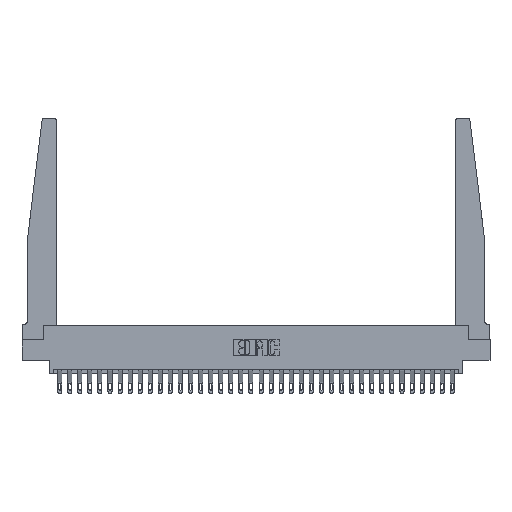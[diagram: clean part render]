
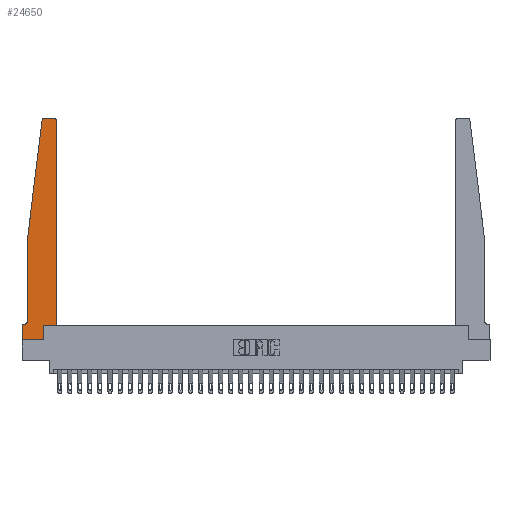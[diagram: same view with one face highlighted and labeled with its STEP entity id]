
A CAD part, top view. The second image highlights one B-rep face of the part: STEP entity #24650.
In plain terms, the highlighted planar face has unit normal (0, 0, 1).
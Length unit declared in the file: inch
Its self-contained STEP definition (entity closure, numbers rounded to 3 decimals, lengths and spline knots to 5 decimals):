
#152 = DIRECTION ( 'NONE',  ( 1., 0., 0. ) ) ;
#312 = PLANE ( 'NONE',  #7482 ) ;
#582 = CARTESIAN_POINT ( 'NONE',  ( 0.065, 1.25, 0.37 ) ) ;
#1792 = ORIENTED_EDGE ( 'NONE', *, *, #31335, .T. ) ;
#2020 = ORIENTED_EDGE ( 'NONE', *, *, #15700, .T. ) ;
#2259 = VECTOR ( 'NONE', #19090, 39.37008 ) ;
#2530 = DIRECTION ( 'NONE',  ( -1., 0., 0. ) ) ;
#2565 = VERTEX_POINT ( 'NONE', #5138 ) ;
#3708 = DIRECTION ( 'NONE',  ( 0., 0., 1. ) ) ;
#4409 = ORIENTED_EDGE ( 'NONE', *, *, #10294, .T. ) ;
#4906 = CIRCLE ( 'NONE', #15784, 0.03 ) ;
#4925 = EDGE_LOOP ( 'NONE', ( #30209, #31184, #9710, #9682, #20174, #4409, #19784, #1792, #2020, #24853, #12709, #20720 ) ) ;
#5138 = CARTESIAN_POINT ( 'NONE',  ( 0.2605, 0.18, 0.37 ) ) ;
#5586 = CARTESIAN_POINT ( 'NONE',  ( 0.425, 0.18, 0.37 ) ) ;
#5610 = CARTESIAN_POINT ( 'NONE',  ( 0.015, 0.2375, 0.37 ) ) ;
#5785 = DIRECTION ( 'NONE',  ( 0., -1., 0. ) ) ;
#7321 = CARTESIAN_POINT ( 'NONE',  ( 0., 0., 0.37 ) ) ;
#7384 = DIRECTION ( 'NONE',  ( 0., 1., 0. ) ) ;
#7482 = AXIS2_PLACEMENT_3D ( 'NONE', #13134, #24829, #152 ) ;
#7746 = VECTOR ( 'NONE', #2530, 39.37008 ) ;
#8170 = EDGE_CURVE ( 'NONE', #2565, #14448, #26695, .T. ) ;
#9081 = VERTEX_POINT ( 'NONE', #29151 ) ;
#9682 = ORIENTED_EDGE ( 'NONE', *, *, #30110, .T. ) ;
#9704 = EDGE_CURVE ( 'NONE', #14448, #24327, #17761, .T. ) ;
#9710 = ORIENTED_EDGE ( 'NONE', *, *, #24084, .T. ) ;
#9741 = EDGE_CURVE ( 'NONE', #17023, #22354, #15329, .T. ) ;
#9777 = VECTOR ( 'NONE', #9955, 39.37008 ) ;
#9955 = DIRECTION ( 'NONE',  ( 0., -1., 0. ) ) ;
#10294 = EDGE_CURVE ( 'NONE', #11463, #24770, #20957, .T. ) ;
#10529 = CARTESIAN_POINT ( 'NONE',  ( 0.24675, 2.72367, 0.37 ) ) ;
#10825 = CARTESIAN_POINT ( 'NONE',  ( 0.065, 1.25, 0.37 ) ) ;
#10858 = CARTESIAN_POINT ( 'NONE',  ( 0., 0.1875, 0.37 ) ) ;
#11349 = VECTOR ( 'NONE', #27652, 39.37008 ) ;
#11463 = VERTEX_POINT ( 'NONE', #30847 ) ;
#11515 = VECTOR ( 'NONE', #7384, 39.37008 ) ;
#11937 = DIRECTION ( 'NONE',  ( 0., 0., 1. ) ) ;
#11976 = CARTESIAN_POINT ( 'NONE',  ( 0., 0., 0.37 ) ) ;
#12094 = CARTESIAN_POINT ( 'NONE',  ( 0.395, 2.72, 0.37 ) ) ;
#12186 = DIRECTION ( 'NONE',  ( 1., 0., 0. ) ) ;
#12709 = ORIENTED_EDGE ( 'NONE', *, *, #9704, .T. ) ;
#13134 = CARTESIAN_POINT ( 'NONE',  ( 0., 0.1875, 0.37 ) ) ;
#13594 = AXIS2_PLACEMENT_3D ( 'NONE', #5610, #17783, #27669 ) ;
#13626 = DIRECTION ( 'NONE',  ( 1., 0., 0. ) ) ;
#14052 = DIRECTION ( 'NONE',  ( 1., 0., 0. ) ) ;
#14448 = VERTEX_POINT ( 'NONE', #26674 ) ;
#14480 = VECTOR ( 'NONE', #28961, 39.37008 ) ;
#14578 = EDGE_CURVE ( 'NONE', #24770, #17082, #29259, .T. ) ;
#15088 = FACE_OUTER_BOUND ( 'NONE', #4925, .T. ) ;
#15329 = LINE ( 'NONE', #24750, #7746 ) ;
#15700 = EDGE_CURVE ( 'NONE', #9081, #2565, #24905, .T. ) ;
#15784 = AXIS2_PLACEMENT_3D ( 'NONE', #12094, #11937, #14052 ) ;
#16792 = CARTESIAN_POINT ( 'NONE',  ( 0.425, 0.18, 0.37 ) ) ;
#16940 = CARTESIAN_POINT ( 'NONE',  ( 0., 0., 0.37 ) ) ;
#17023 = VERTEX_POINT ( 'NONE', #29014 ) ;
#17082 = VERTEX_POINT ( 'NONE', #11976 ) ;
#17761 = LINE ( 'NONE', #5586, #11349 ) ;
#17783 = DIRECTION ( 'NONE',  ( 0., 0., -1. ) ) ;
#17873 = EDGE_CURVE ( 'NONE', #26345, #11463, #24472, .T. ) ;
#18444 = CARTESIAN_POINT ( 'NONE',  ( 0.065, 0.2375, 0.37 ) ) ;
#18525 = CARTESIAN_POINT ( 'NONE',  ( 0.065, 0.1875, 0.37 ) ) ;
#18791 = CARTESIAN_POINT ( 'NONE',  ( 0.27653, 2.75, 0.37 ) ) ;
#18938 = EDGE_CURVE ( 'NONE', #22354, #28500, #23054, .T. ) ;
#19090 = DIRECTION ( 'NONE',  ( -0.122, -0.992, 0. ) ) ;
#19181 = LINE ( 'NONE', #7321, #20954 ) ;
#19784 = ORIENTED_EDGE ( 'NONE', *, *, #14578, .T. ) ;
#20174 = ORIENTED_EDGE ( 'NONE', *, *, #17873, .T. ) ;
#20720 = ORIENTED_EDGE ( 'NONE', *, *, #25267, .T. ) ;
#20904 = VECTOR ( 'NONE', #5785, 39.37008 ) ;
#20954 = VECTOR ( 'NONE', #12186, 39.37008 ) ;
#20957 = LINE ( 'NONE', #18525, #27444 ) ;
#20992 = CARTESIAN_POINT ( 'NONE',  ( 0.425, 2.72, 0.37 ) ) ;
#21817 = CARTESIAN_POINT ( 'NONE',  ( 0.2605, 0.18, 0.37 ) ) ;
#22354 = VERTEX_POINT ( 'NONE', #18791 ) ;
#23054 = CIRCLE ( 'NONE', #27200, 0.03 ) ;
#24084 = EDGE_CURVE ( 'NONE', #28500, #30080, #30748, .T. ) ;
#24327 = VERTEX_POINT ( 'NONE', #20992 ) ;
#24472 = CIRCLE ( 'NONE', #13594, 0.05 ) ;
#24650 = ADVANCED_FACE ( 'NONE', ( #15088 ), #312, .T. ) ;
#24750 = CARTESIAN_POINT ( 'NONE',  ( 0.25, 2.75, 0.37 ) ) ;
#24770 = VERTEX_POINT ( 'NONE', #10858 ) ;
#24829 = DIRECTION ( 'NONE',  ( 0., 0., 1. ) ) ;
#24853 = ORIENTED_EDGE ( 'NONE', *, *, #8170, .T. ) ;
#24905 = LINE ( 'NONE', #21817, #11515 ) ;
#25267 = EDGE_CURVE ( 'NONE', #24327, #17023, #4906, .T. ) ;
#25955 = CARTESIAN_POINT ( 'NONE',  ( 0.27653, 2.72, 0.37 ) ) ;
#26345 = VERTEX_POINT ( 'NONE', #18444 ) ;
#26674 = CARTESIAN_POINT ( 'NONE',  ( 0.425, 0.18, 0.37 ) ) ;
#26695 = LINE ( 'NONE', #16792, #14480 ) ;
#27200 = AXIS2_PLACEMENT_3D ( 'NONE', #25955, #3708, #13626 ) ;
#27444 = VECTOR ( 'NONE', #30520, 39.37008 ) ;
#27652 = DIRECTION ( 'NONE',  ( 0., 1., 0. ) ) ;
#27669 = DIRECTION ( 'NONE',  ( -1., 0., 0. ) ) ;
#28169 = LINE ( 'NONE', #10825, #20904 ) ;
#28500 = VERTEX_POINT ( 'NONE', #10529 ) ;
#28961 = DIRECTION ( 'NONE',  ( 1., 0., 0. ) ) ;
#29014 = CARTESIAN_POINT ( 'NONE',  ( 0.395, 2.75, 0.37 ) ) ;
#29151 = CARTESIAN_POINT ( 'NONE',  ( 0.2605, 0., 0.37 ) ) ;
#29259 = LINE ( 'NONE', #16940, #9777 ) ;
#30080 = VERTEX_POINT ( 'NONE', #582 ) ;
#30110 = EDGE_CURVE ( 'NONE', #30080, #26345, #28169, .T. ) ;
#30209 = ORIENTED_EDGE ( 'NONE', *, *, #9741, .T. ) ;
#30520 = DIRECTION ( 'NONE',  ( -1., 0., 0. ) ) ;
#30748 = LINE ( 'NONE', #31080, #2259 ) ;
#30847 = CARTESIAN_POINT ( 'NONE',  ( 0.015, 0.1875, 0.37 ) ) ;
#31080 = CARTESIAN_POINT ( 'NONE',  ( 0.065, 1.25, 0.37 ) ) ;
#31184 = ORIENTED_EDGE ( 'NONE', *, *, #18938, .T. ) ;
#31335 = EDGE_CURVE ( 'NONE', #17082, #9081, #19181, .T. ) ;
